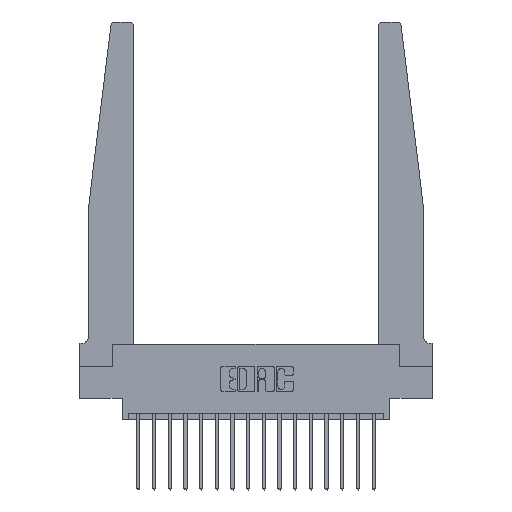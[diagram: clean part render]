
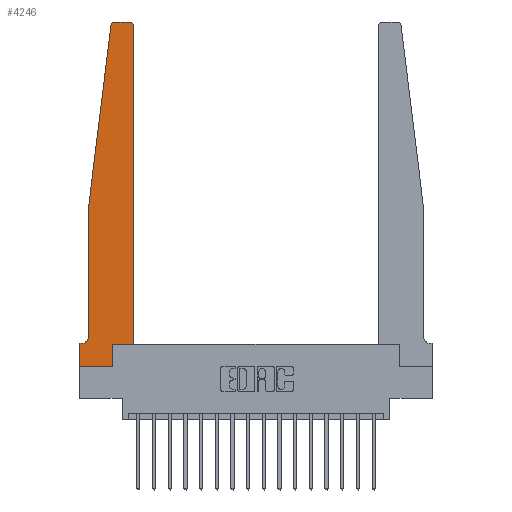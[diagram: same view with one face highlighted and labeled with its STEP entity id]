
A CAD part, top view. The second image highlights one B-rep face of the part: STEP entity #4246.
In plain terms, the highlighted planar face has unit normal (0, 0, 1).
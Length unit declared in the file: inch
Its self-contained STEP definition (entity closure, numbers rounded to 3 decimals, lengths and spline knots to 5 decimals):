
#128 = DIRECTION ( 'NONE',  ( 0., 1., 0. ) ) ;
#320 = EDGE_CURVE ( 'NONE', #8806, #1453, #5530, .T. ) ;
#339 = EDGE_CURVE ( 'NONE', #15717, #9029, #11480, .T. ) ;
#454 = CARTESIAN_POINT ( 'NONE',  ( 0.065, 1.25, 0.37 ) ) ;
#500 = EDGE_CURVE ( 'NONE', #7259, #9388, #10623, .T. ) ;
#514 = VECTOR ( 'NONE', #737, 39.37008 ) ;
#570 = CARTESIAN_POINT ( 'NONE',  ( 0.425, 0.18, 0.37 ) ) ;
#723 = VERTEX_POINT ( 'NONE', #4928 ) ;
#737 = DIRECTION ( 'NONE',  ( 1., 0., 0. ) ) ;
#1001 = FACE_OUTER_BOUND ( 'NONE', #16033, .T. ) ;
#1130 = DIRECTION ( 'NONE',  ( 0., -1., 0. ) ) ;
#1220 = EDGE_CURVE ( 'NONE', #723, #3827, #9568, .T. ) ;
#1449 = VERTEX_POINT ( 'NONE', #12473 ) ;
#1453 = VERTEX_POINT ( 'NONE', #18455 ) ;
#2103 = VERTEX_POINT ( 'NONE', #18127 ) ;
#2293 = ORIENTED_EDGE ( 'NONE', *, *, #12915, .T. ) ;
#2295 = CIRCLE ( 'NONE', #5428, 0.05 ) ;
#2317 = CARTESIAN_POINT ( 'NONE',  ( 0.065, 0.2375, 0.37 ) ) ;
#3351 = CARTESIAN_POINT ( 'NONE',  ( 0.065, 1.25, 0.37 ) ) ;
#3484 = DIRECTION ( 'NONE',  ( 1., 0., 0. ) ) ;
#3827 = VERTEX_POINT ( 'NONE', #11417 ) ;
#4246 = ADVANCED_FACE ( 'NONE', ( #1001 ), #8591, .T. ) ;
#4319 = DIRECTION ( 'NONE',  ( 1., 0., 0. ) ) ;
#4526 = CARTESIAN_POINT ( 'NONE',  ( 0.2605, 0.18, 0.37 ) ) ;
#4845 = VECTOR ( 'NONE', #15606, 39.37008 ) ;
#4928 = CARTESIAN_POINT ( 'NONE',  ( 0.2605, 0.18, 0.37 ) ) ;
#5383 = DIRECTION ( 'NONE',  ( -1., 0., 0. ) ) ;
#5428 = AXIS2_PLACEMENT_3D ( 'NONE', #11604, #10037, #5383 ) ;
#5530 = LINE ( 'NONE', #14237, #6093 ) ;
#5620 = LINE ( 'NONE', #9604, #4845 ) ;
#5668 = EDGE_CURVE ( 'NONE', #1449, #15717, #5620, .T. ) ;
#6086 = LINE ( 'NONE', #4526, #18372 ) ;
#6093 = VECTOR ( 'NONE', #7186, 39.37008 ) ;
#6411 = EDGE_CURVE ( 'NONE', #3827, #2103, #13955, .T. ) ;
#6819 = EDGE_CURVE ( 'NONE', #9029, #13793, #15613, .T. ) ;
#6944 = ORIENTED_EDGE ( 'NONE', *, *, #18312, .T. ) ;
#7087 = ORIENTED_EDGE ( 'NONE', *, *, #320, .T. ) ;
#7186 = DIRECTION ( 'NONE',  ( -1., 0., 0. ) ) ;
#7230 = CARTESIAN_POINT ( 'NONE',  ( 0.065, 1.25, 0.37 ) ) ;
#7259 = VERTEX_POINT ( 'NONE', #18990 ) ;
#8422 = CIRCLE ( 'NONE', #11183, 0.03 ) ;
#8591 = PLANE ( 'NONE',  #12755 ) ;
#8706 = DIRECTION ( 'NONE',  ( 0., 0., 1. ) ) ;
#8806 = VERTEX_POINT ( 'NONE', #18447 ) ;
#9029 = VERTEX_POINT ( 'NONE', #18824 ) ;
#9058 = EDGE_CURVE ( 'NONE', #13793, #723, #6086, .T. ) ;
#9090 = CARTESIAN_POINT ( 'NONE',  ( 0.2605, 0., 0.37 ) ) ;
#9233 = CARTESIAN_POINT ( 'NONE',  ( 0.27653, 2.72, 0.37 ) ) ;
#9384 = LINE ( 'NONE', #3351, #18521 ) ;
#9388 = VERTEX_POINT ( 'NONE', #7230 ) ;
#9568 = LINE ( 'NONE', #15771, #14016 ) ;
#9604 = CARTESIAN_POINT ( 'NONE',  ( 0.065, 0.1875, 0.37 ) ) ;
#10037 = DIRECTION ( 'NONE',  ( 0., 0., -1. ) ) ;
#10623 = LINE ( 'NONE', #454, #18664 ) ;
#10704 = ORIENTED_EDGE ( 'NONE', *, *, #1220, .T. ) ;
#11091 = VECTOR ( 'NONE', #17112, 39.37008 ) ;
#11183 = AXIS2_PLACEMENT_3D ( 'NONE', #9233, #15225, #3484 ) ;
#11294 = VERTEX_POINT ( 'NONE', #2317 ) ;
#11417 = CARTESIAN_POINT ( 'NONE',  ( 0.425, 0.18, 0.37 ) ) ;
#11480 = LINE ( 'NONE', #14524, #17061 ) ;
#11483 = ORIENTED_EDGE ( 'NONE', *, *, #14476, .T. ) ;
#11518 = DIRECTION ( 'NONE',  ( 1., 0., 0. ) ) ;
#11604 = CARTESIAN_POINT ( 'NONE',  ( 0.015, 0.2375, 0.37 ) ) ;
#12061 = ORIENTED_EDGE ( 'NONE', *, *, #6819, .T. ) ;
#12473 = CARTESIAN_POINT ( 'NONE',  ( 0.015, 0.1875, 0.37 ) ) ;
#12755 = AXIS2_PLACEMENT_3D ( 'NONE', #12821, #8706, #4319 ) ;
#12821 = CARTESIAN_POINT ( 'NONE',  ( 0., 0.1875, 0.37 ) ) ;
#12887 = ORIENTED_EDGE ( 'NONE', *, *, #6411, .T. ) ;
#12915 = EDGE_CURVE ( 'NONE', #1453, #7259, #8422, .T. ) ;
#12989 = ORIENTED_EDGE ( 'NONE', *, *, #500, .T. ) ;
#13092 = DIRECTION ( 'NONE',  ( 0., 0., 1. ) ) ;
#13098 = CARTESIAN_POINT ( 'NONE',  ( 0., 0.1875, 0.37 ) ) ;
#13793 = VERTEX_POINT ( 'NONE', #9090 ) ;
#13883 = DIRECTION ( 'NONE',  ( 1., 0., 0. ) ) ;
#13955 = LINE ( 'NONE', #570, #11091 ) ;
#14016 = VECTOR ( 'NONE', #13883, 39.37008 ) ;
#14237 = CARTESIAN_POINT ( 'NONE',  ( 0.25, 2.75, 0.37 ) ) ;
#14476 = EDGE_CURVE ( 'NONE', #11294, #1449, #2295, .T. ) ;
#14524 = CARTESIAN_POINT ( 'NONE',  ( 0., 0., 0.37 ) ) ;
#14560 = ORIENTED_EDGE ( 'NONE', *, *, #14985, .T. ) ;
#14571 = AXIS2_PLACEMENT_3D ( 'NONE', #15653, #13092, #11518 ) ;
#14985 = EDGE_CURVE ( 'NONE', #9388, #11294, #9384, .T. ) ;
#15225 = DIRECTION ( 'NONE',  ( 0., 0., 1. ) ) ;
#15401 = CARTESIAN_POINT ( 'NONE',  ( 0., 0., 0.37 ) ) ;
#15606 = DIRECTION ( 'NONE',  ( -1., 0., 0. ) ) ;
#15613 = LINE ( 'NONE', #15401, #514 ) ;
#15653 = CARTESIAN_POINT ( 'NONE',  ( 0.395, 2.72, 0.37 ) ) ;
#15717 = VERTEX_POINT ( 'NONE', #13098 ) ;
#15771 = CARTESIAN_POINT ( 'NONE',  ( 0.425, 0.18, 0.37 ) ) ;
#16033 = EDGE_LOOP ( 'NONE', ( #7087, #2293, #12989, #14560, #11483, #19053, #17431, #12061, #17405, #10704, #12887, #6944 ) ) ;
#16769 = DIRECTION ( 'NONE',  ( 0., -1., 0. ) ) ;
#16825 = DIRECTION ( 'NONE',  ( -0.122, -0.992, 0. ) ) ;
#17061 = VECTOR ( 'NONE', #1130, 39.37008 ) ;
#17112 = DIRECTION ( 'NONE',  ( 0., 1., 0. ) ) ;
#17405 = ORIENTED_EDGE ( 'NONE', *, *, #9058, .T. ) ;
#17431 = ORIENTED_EDGE ( 'NONE', *, *, #339, .T. ) ;
#18127 = CARTESIAN_POINT ( 'NONE',  ( 0.425, 2.72, 0.37 ) ) ;
#18312 = EDGE_CURVE ( 'NONE', #2103, #8806, #18626, .T. ) ;
#18372 = VECTOR ( 'NONE', #128, 39.37008 ) ;
#18447 = CARTESIAN_POINT ( 'NONE',  ( 0.395, 2.75, 0.37 ) ) ;
#18455 = CARTESIAN_POINT ( 'NONE',  ( 0.27653, 2.75, 0.37 ) ) ;
#18521 = VECTOR ( 'NONE', #16769, 39.37008 ) ;
#18626 = CIRCLE ( 'NONE', #14571, 0.03 ) ;
#18664 = VECTOR ( 'NONE', #16825, 39.37008 ) ;
#18824 = CARTESIAN_POINT ( 'NONE',  ( 0., 0., 0.37 ) ) ;
#18990 = CARTESIAN_POINT ( 'NONE',  ( 0.24675, 2.72367, 0.37 ) ) ;
#19053 = ORIENTED_EDGE ( 'NONE', *, *, #5668, .T. ) ;
